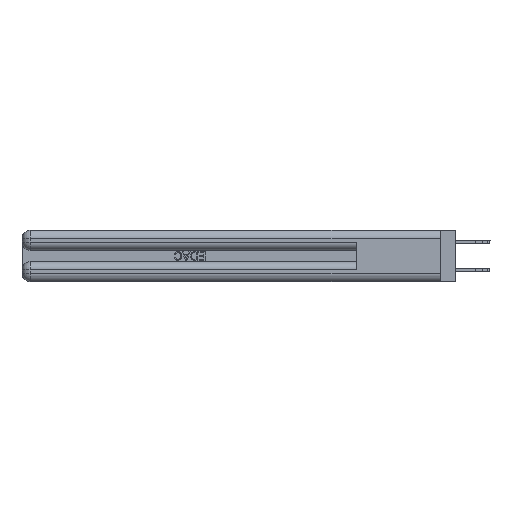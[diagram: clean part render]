
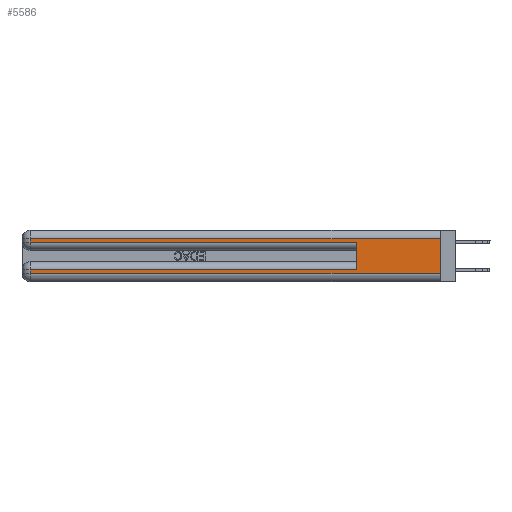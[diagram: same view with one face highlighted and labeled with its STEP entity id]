
A CAD part, left-side view. The second image highlights one B-rep face of the part: STEP entity #5586.
In plain terms, the highlighted planar face has unit normal (-1, 0, 0).
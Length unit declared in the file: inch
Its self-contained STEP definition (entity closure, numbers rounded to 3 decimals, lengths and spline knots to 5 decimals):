
#222 = VECTOR ( 'NONE', #25706, 39.37008 ) ;
#244 = VERTEX_POINT ( 'NONE', #19764 ) ;
#332 = VERTEX_POINT ( 'NONE', #7213 ) ;
#507 = CARTESIAN_POINT ( 'NONE',  ( 0., 0., 0.31 ) ) ;
#949 = CARTESIAN_POINT ( 'NONE',  ( 0., 2.94, 0.06 ) ) ;
#994 = EDGE_CURVE ( 'NONE', #244, #26739, #12634, .T. ) ;
#1316 = CARTESIAN_POINT ( 'NONE',  ( 0., 2.94, 0.37 ) ) ;
#1456 = CARTESIAN_POINT ( 'NONE',  ( 0., 0.6, 0.285 ) ) ;
#1648 = ORIENTED_EDGE ( 'NONE', *, *, #13724, .F. ) ;
#2831 = VERTEX_POINT ( 'NONE', #507 ) ;
#3841 = VECTOR ( 'NONE', #33147, 39.37008 ) ;
#5083 = LINE ( 'NONE', #17426, #5587 ) ;
#5586 = ADVANCED_FACE ( 'NONE', ( #37124 ), #29228, .F. ) ;
#5587 = VECTOR ( 'NONE', #14588, 39.37008 ) ;
#5610 = CARTESIAN_POINT ( 'NONE',  ( 0., 2.94, 0.31 ) ) ;
#6508 = EDGE_CURVE ( 'NONE', #2831, #332, #16300, .T. ) ;
#6616 = VECTOR ( 'NONE', #10067, 39.37008 ) ;
#6823 = AXIS2_PLACEMENT_3D ( 'NONE', #7518, #38043, #10984 ) ;
#7213 = CARTESIAN_POINT ( 'NONE',  ( 0., 0., 0.06 ) ) ;
#7518 = CARTESIAN_POINT ( 'NONE',  ( 0., 0., 0.37 ) ) ;
#8414 = DIRECTION ( 'NONE',  ( 0., 1., 0. ) ) ;
#8436 = VERTEX_POINT ( 'NONE', #21994 ) ;
#8885 = VECTOR ( 'NONE', #26872, 39.37008 ) ;
#10067 = DIRECTION ( 'NONE',  ( 0., 0., -1. ) ) ;
#10312 = ORIENTED_EDGE ( 'NONE', *, *, #31142, .T. ) ;
#10984 = DIRECTION ( 'NONE',  ( 0., 0., -1. ) ) ;
#11617 = VERTEX_POINT ( 'NONE', #34367 ) ;
#12634 = LINE ( 'NONE', #16989, #8885 ) ;
#13724 = EDGE_CURVE ( 'NONE', #11617, #26739, #16621, .T. ) ;
#14588 = DIRECTION ( 'NONE',  ( 0., 1., 0. ) ) ;
#15305 = LINE ( 'NONE', #32514, #29187 ) ;
#16300 = LINE ( 'NONE', #31409, #23951 ) ;
#16621 = LINE ( 'NONE', #31830, #33385 ) ;
#16974 = ORIENTED_EDGE ( 'NONE', *, *, #24064, .T. ) ;
#16989 = CARTESIAN_POINT ( 'NONE',  ( 0., 0., 0.285 ) ) ;
#17426 = CARTESIAN_POINT ( 'NONE',  ( 0., 0., 0.31 ) ) ;
#18791 = VERTEX_POINT ( 'NONE', #949 ) ;
#19409 = DIRECTION ( 'NONE',  ( 0., 0., -1. ) ) ;
#19764 = CARTESIAN_POINT ( 'NONE',  ( 0., 2.94, 0.285 ) ) ;
#20189 = ORIENTED_EDGE ( 'NONE', *, *, #27554, .T. ) ;
#20655 = ORIENTED_EDGE ( 'NONE', *, *, #994, .T. ) ;
#21994 = CARTESIAN_POINT ( 'NONE',  ( 0., 2.94, 0.085 ) ) ;
#23951 = VECTOR ( 'NONE', #19409, 39.37008 ) ;
#24064 = EDGE_CURVE ( 'NONE', #8436, #18791, #33357, .T. ) ;
#24466 = CARTESIAN_POINT ( 'NONE',  ( 0., 0., 0.06 ) ) ;
#25222 = ORIENTED_EDGE ( 'NONE', *, *, #26906, .T. ) ;
#25382 = CARTESIAN_POINT ( 'NONE',  ( 0., 2.94, 0.37 ) ) ;
#25566 = EDGE_CURVE ( 'NONE', #2831, #31500, #5083, .T. ) ;
#25706 = DIRECTION ( 'NONE',  ( 0., 0., -1. ) ) ;
#26439 = ORIENTED_EDGE ( 'NONE', *, *, #25566, .T. ) ;
#26739 = VERTEX_POINT ( 'NONE', #1456 ) ;
#26872 = DIRECTION ( 'NONE',  ( 0., -1., 0. ) ) ;
#26906 = EDGE_CURVE ( 'NONE', #11617, #8436, #15305, .T. ) ;
#27554 = EDGE_CURVE ( 'NONE', #18791, #332, #34365, .T. ) ;
#29187 = VECTOR ( 'NONE', #8414, 39.37008 ) ;
#29228 = PLANE ( 'NONE',  #6823 ) ;
#31142 = EDGE_CURVE ( 'NONE', #31500, #244, #35059, .T. ) ;
#31409 = CARTESIAN_POINT ( 'NONE',  ( 0., 0., 0.37 ) ) ;
#31500 = VERTEX_POINT ( 'NONE', #5610 ) ;
#31830 = CARTESIAN_POINT ( 'NONE',  ( 0., 0.6, 0.145 ) ) ;
#32514 = CARTESIAN_POINT ( 'NONE',  ( 0., 0., 0.085 ) ) ;
#33108 = EDGE_LOOP ( 'NONE', ( #34208, #26439, #10312, #20655, #1648, #25222, #16974, #20189 ) ) ;
#33147 = DIRECTION ( 'NONE',  ( 0., -1., 0. ) ) ;
#33357 = LINE ( 'NONE', #25382, #6616 ) ;
#33385 = VECTOR ( 'NONE', #34787, 39.37008 ) ;
#34208 = ORIENTED_EDGE ( 'NONE', *, *, #6508, .F. ) ;
#34365 = LINE ( 'NONE', #24466, #3841 ) ;
#34367 = CARTESIAN_POINT ( 'NONE',  ( 0., 0.6, 0.085 ) ) ;
#34787 = DIRECTION ( 'NONE',  ( 0., 0., 1. ) ) ;
#35059 = LINE ( 'NONE', #1316, #222 ) ;
#37124 = FACE_OUTER_BOUND ( 'NONE', #33108, .T. ) ;
#38043 = DIRECTION ( 'NONE',  ( 1., 0., 0. ) ) ;
